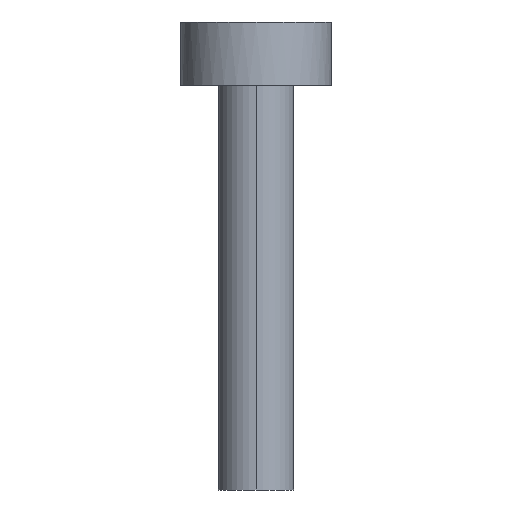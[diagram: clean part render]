
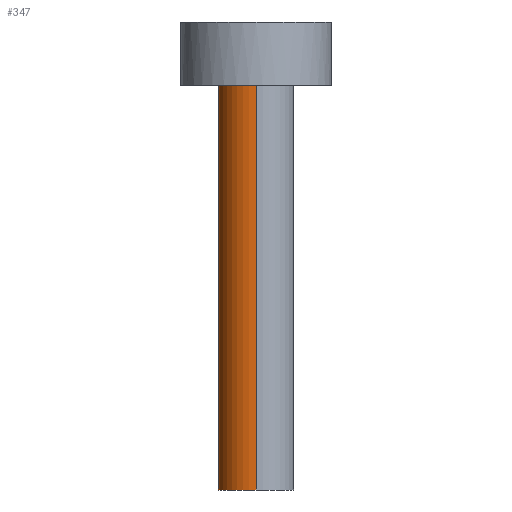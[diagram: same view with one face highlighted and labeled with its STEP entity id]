
A CAD part, left-side view. The second image highlights one B-rep face of the part: STEP entity #347.
In plain terms, the highlighted cylindrical face has radius 3 mm (diameter 6 mm), a partial arc.
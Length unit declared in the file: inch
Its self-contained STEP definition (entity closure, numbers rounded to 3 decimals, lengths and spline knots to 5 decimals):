
#52 = DIRECTION ( 'NONE',  ( -1., 0., 0. ) ) ;
#54 = ORIENTED_EDGE ( 'NONE', *, *, #459, .T. ) ;
#71 = DIRECTION ( 'NONE',  ( 0., 0., -1. ) ) ;
#81 = ORIENTED_EDGE ( 'NONE', *, *, #452, .F. ) ;
#141 = CARTESIAN_POINT ( 'NONE',  ( -4.95254, -0.47191, -1.26378 ) ) ;
#204 = CARTESIAN_POINT ( 'NONE',  ( -4.83443, -0.47191, 0.19685 ) ) ;
#219 = CARTESIAN_POINT ( 'NONE',  ( -4.83443, -0.47191, -1.26378 ) ) ;
#270 = VERTEX_POINT ( 'NONE', #874 ) ;
#279 = ORIENTED_EDGE ( 'NONE', *, *, #450, .F. ) ;
#295 = DIRECTION ( 'NONE',  ( -1., 0., 0. ) ) ;
#296 = AXIS2_PLACEMENT_3D ( 'NONE', #219, #731, #295 ) ;
#304 = AXIS2_PLACEMENT_3D ( 'NONE', #520, #71, #592 ) ;
#335 = AXIS2_PLACEMENT_3D ( 'NONE', #204, #506, #52 ) ;
#347 = ADVANCED_FACE ( 'NONE', ( #804 ), #785, .T. ) ;
#402 = VERTEX_POINT ( 'NONE', #584 ) ;
#444 = DIRECTION ( 'NONE',  ( 0., 0., -1. ) ) ;
#450 = EDGE_CURVE ( 'NONE', #270, #596, #842, .T. ) ;
#452 = EDGE_CURVE ( 'NONE', #596, #876, #505, .T. ) ;
#456 = ORIENTED_EDGE ( 'NONE', *, *, #465, .T. ) ;
#459 = EDGE_CURVE ( 'NONE', #402, #876, #702, .T. ) ;
#465 = EDGE_CURVE ( 'NONE', #270, #402, #826, .T. ) ;
#505 = CIRCLE ( 'NONE', #296, 0.11811 ) ;
#506 = DIRECTION ( 'NONE',  ( 0., 0., -1. ) ) ;
#519 = DIRECTION ( 'NONE',  ( 0., 0., -1. ) ) ;
#520 = CARTESIAN_POINT ( 'NONE',  ( -4.83443, -0.47191, 0. ) ) ;
#584 = CARTESIAN_POINT ( 'NONE',  ( -4.71632, -0.47191, 0. ) ) ;
#592 = DIRECTION ( 'NONE',  ( -1., 0., 0. ) ) ;
#596 = VERTEX_POINT ( 'NONE', #141 ) ;
#671 = CARTESIAN_POINT ( 'NONE',  ( -4.71632, -0.47191, 0.19685 ) ) ;
#684 = VECTOR ( 'NONE', #444, 39.37008 ) ;
#702 = LINE ( 'NONE', #671, #684 ) ;
#714 = VECTOR ( 'NONE', #519, 39.37008 ) ;
#731 = DIRECTION ( 'NONE',  ( 0., 0., -1. ) ) ;
#777 = CARTESIAN_POINT ( 'NONE',  ( -4.95254, -0.47191, 0.19685 ) ) ;
#785 = CYLINDRICAL_SURFACE ( 'NONE', #335, 0.11811 ) ;
#804 = FACE_OUTER_BOUND ( 'NONE', #849, .T. ) ;
#826 = CIRCLE ( 'NONE', #304, 0.11811 ) ;
#842 = LINE ( 'NONE', #777, #714 ) ;
#849 = EDGE_LOOP ( 'NONE', ( #456, #54, #81, #279 ) ) ;
#859 = CARTESIAN_POINT ( 'NONE',  ( -4.71632, -0.47191, -1.26378 ) ) ;
#874 = CARTESIAN_POINT ( 'NONE',  ( -4.95254, -0.47191, 0. ) ) ;
#876 = VERTEX_POINT ( 'NONE', #859 ) ;
